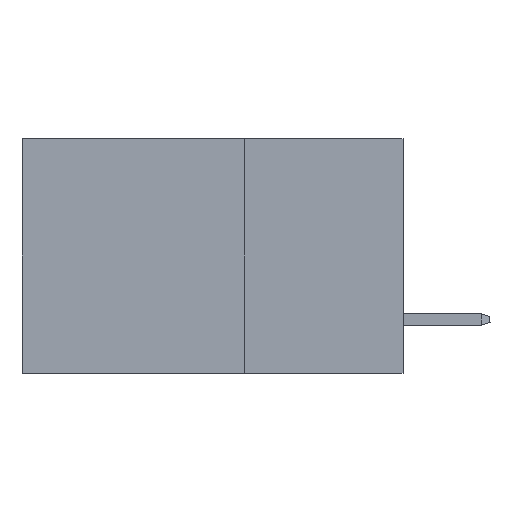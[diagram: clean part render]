
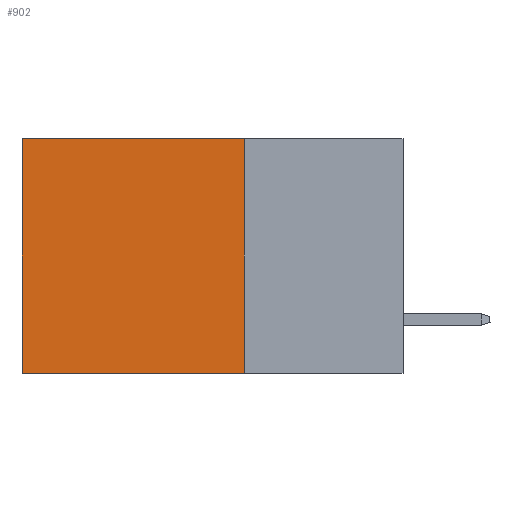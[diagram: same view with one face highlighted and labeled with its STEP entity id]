
A CAD part, left-side view. The second image highlights one B-rep face of the part: STEP entity #902.
In plain terms, the highlighted planar face has unit normal (-1, 0, 0).
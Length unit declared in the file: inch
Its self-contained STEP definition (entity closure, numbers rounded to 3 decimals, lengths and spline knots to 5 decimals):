
#605 = DIRECTION ( 'NONE',  ( 0., 0., -1. ) ) ;
#632 = LINE ( 'NONE', #14118, #2678 ) ;
#729 = CARTESIAN_POINT ( 'NONE',  ( 0.2875, 0.25, -0.37 ) ) ;
#785 = CARTESIAN_POINT ( 'NONE',  ( 0.2875, 0.25, 0. ) ) ;
#902 = ADVANCED_FACE ( 'NONE', ( #17725 ), #1805, .F. ) ;
#1805 = PLANE ( 'NONE',  #7725 ) ;
#1968 = VECTOR ( 'NONE', #6404, 39.37008 ) ;
#2166 = VERTEX_POINT ( 'NONE', #4537 ) ;
#2364 = VECTOR ( 'NONE', #15273, 39.37008 ) ;
#2556 = EDGE_LOOP ( 'NONE', ( #9679, #3061, #4188, #8216 ) ) ;
#2678 = VECTOR ( 'NONE', #17029, 39.37008 ) ;
#3061 = ORIENTED_EDGE ( 'NONE', *, *, #3393, .F. ) ;
#3351 = DIRECTION ( 'NONE',  ( 1., 0., 0. ) ) ;
#3393 = EDGE_CURVE ( 'NONE', #5305, #18461, #7138, .T. ) ;
#3601 = CARTESIAN_POINT ( 'NONE',  ( 0.2875, 0.25, 0. ) ) ;
#4188 = ORIENTED_EDGE ( 'NONE', *, *, #15837, .F. ) ;
#4537 = CARTESIAN_POINT ( 'NONE',  ( 0.2875, 0.6, 0. ) ) ;
#5305 = VERTEX_POINT ( 'NONE', #729 ) ;
#5392 = LINE ( 'NONE', #785, #2364 ) ;
#5866 = VERTEX_POINT ( 'NONE', #16066 ) ;
#6404 = DIRECTION ( 'NONE',  ( 0., 1., 0. ) ) ;
#7138 = LINE ( 'NONE', #15753, #8292 ) ;
#7725 = AXIS2_PLACEMENT_3D ( 'NONE', #14796, #3351, #605 ) ;
#8216 = ORIENTED_EDGE ( 'NONE', *, *, #12618, .T. ) ;
#8292 = VECTOR ( 'NONE', #8588, 39.37008 ) ;
#8588 = DIRECTION ( 'NONE',  ( 0., 1., 0. ) ) ;
#9679 = ORIENTED_EDGE ( 'NONE', *, *, #16573, .T. ) ;
#12618 = EDGE_CURVE ( 'NONE', #5866, #2166, #16833, .T. ) ;
#13187 = CARTESIAN_POINT ( 'NONE',  ( 0.2875, 0.6, -0.37 ) ) ;
#14118 = CARTESIAN_POINT ( 'NONE',  ( 0.2875, 0.6, 0. ) ) ;
#14796 = CARTESIAN_POINT ( 'NONE',  ( 0.2875, 0.25, 0. ) ) ;
#15273 = DIRECTION ( 'NONE',  ( 0., 0., -1. ) ) ;
#15753 = CARTESIAN_POINT ( 'NONE',  ( 0.2875, 0.25, -0.37 ) ) ;
#15837 = EDGE_CURVE ( 'NONE', #5866, #5305, #5392, .T. ) ;
#16066 = CARTESIAN_POINT ( 'NONE',  ( 0.2875, 0.25, 0. ) ) ;
#16573 = EDGE_CURVE ( 'NONE', #2166, #18461, #632, .T. ) ;
#16833 = LINE ( 'NONE', #3601, #1968 ) ;
#17029 = DIRECTION ( 'NONE',  ( 0., 0., -1. ) ) ;
#17725 = FACE_OUTER_BOUND ( 'NONE', #2556, .T. ) ;
#18461 = VERTEX_POINT ( 'NONE', #13187 ) ;
